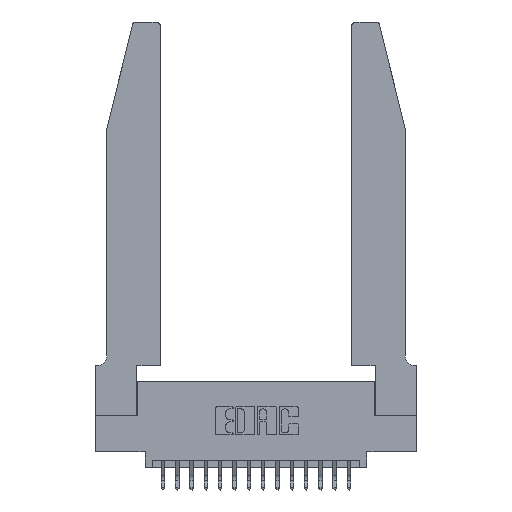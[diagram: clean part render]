
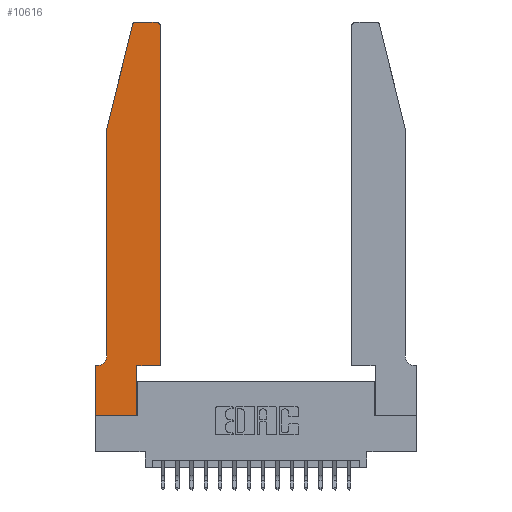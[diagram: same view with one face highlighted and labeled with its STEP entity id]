
A CAD part, top view. The second image highlights one B-rep face of the part: STEP entity #10616.
In plain terms, the highlighted planar face has unit normal (0, 0, 1).
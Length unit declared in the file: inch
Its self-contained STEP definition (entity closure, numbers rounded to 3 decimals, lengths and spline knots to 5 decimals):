
#74 = ORIENTED_EDGE ( 'NONE', *, *, #1063, .T. ) ;
#269 = DIRECTION ( 'NONE',  ( 0., 0., 1. ) ) ;
#299 = VECTOR ( 'NONE', #8002, 39.37008 ) ;
#442 = DIRECTION ( 'NONE',  ( -0.239, -0.971, 0. ) ) ;
#506 = CARTESIAN_POINT ( 'NONE',  ( 0.0755, 2., 0.37 ) ) ;
#681 = CARTESIAN_POINT ( 'NONE',  ( 0.0055, 0.35, 0.37 ) ) ;
#839 = VERTEX_POINT ( 'NONE', #16236 ) ;
#939 = CARTESIAN_POINT ( 'NONE',  ( 0., 0.35, 0.37 ) ) ;
#1063 = EDGE_CURVE ( 'NONE', #10182, #6074, #4686, .T. ) ;
#1089 = DIRECTION ( 'NONE',  ( -1., 0., 0. ) ) ;
#1125 = VECTOR ( 'NONE', #10548, 39.37008 ) ;
#1211 = CARTESIAN_POINT ( 'NONE',  ( 0.4505, 0.35, 0.37 ) ) ;
#1375 = EDGE_CURVE ( 'NONE', #12312, #8913, #15629, .T. ) ;
#1881 = VERTEX_POINT ( 'NONE', #1211 ) ;
#1940 = VECTOR ( 'NONE', #13911, 39.37008 ) ;
#2105 = AXIS2_PLACEMENT_3D ( 'NONE', #9655, #269, #11159 ) ;
#2196 = DIRECTION ( 'NONE',  ( 0., -1., 0. ) ) ;
#2913 = EDGE_CURVE ( 'NONE', #6074, #12196, #3329, .T. ) ;
#3329 = LINE ( 'NONE', #12933, #10999 ) ;
#4033 = CARTESIAN_POINT ( 'NONE',  ( 0.4205, 2.72, 0.37 ) ) ;
#4075 = LINE ( 'NONE', #17051, #299 ) ;
#4520 = DIRECTION ( 'NONE',  ( 0., 0., 1. ) ) ;
#4686 = LINE ( 'NONE', #16599, #12301 ) ;
#4693 = EDGE_LOOP ( 'NONE', ( #14164, #12269, #15600, #19391, #19447, #19095, #74, #7726, #13262, #17609, #11004, #9335 ) ) ;
#5027 = CARTESIAN_POINT ( 'NONE',  ( 0.2865, 0.35, 0.37 ) ) ;
#5591 = DIRECTION ( 'NONE',  ( 1., 0., 0. ) ) ;
#5601 = PLANE ( 'NONE',  #15617 ) ;
#5663 = LINE ( 'NONE', #18467, #1940 ) ;
#5685 = CARTESIAN_POINT ( 'NONE',  ( 0.2865, 0., 0.37 ) ) ;
#5727 = CARTESIAN_POINT ( 'NONE',  ( 0.4505, 0.35, 0.37 ) ) ;
#5868 = CIRCLE ( 'NONE', #13526, 0.03 ) ;
#6023 = CARTESIAN_POINT ( 'NONE',  ( 0.0755, 2., 0.37 ) ) ;
#6074 = VERTEX_POINT ( 'NONE', #13471 ) ;
#6077 = VECTOR ( 'NONE', #15677, 39.37008 ) ;
#6305 = EDGE_CURVE ( 'NONE', #1881, #10761, #5663, .T. ) ;
#7263 = VERTEX_POINT ( 'NONE', #681 ) ;
#7530 = EDGE_CURVE ( 'NONE', #15201, #16020, #12965, .T. ) ;
#7726 = ORIENTED_EDGE ( 'NONE', *, *, #2913, .T. ) ;
#8002 = DIRECTION ( 'NONE',  ( -1., 0., 0. ) ) ;
#8242 = EDGE_CURVE ( 'NONE', #12196, #8375, #17216, .T. ) ;
#8282 = VECTOR ( 'NONE', #442, 39.37008 ) ;
#8375 = VERTEX_POINT ( 'NONE', #14748 ) ;
#8755 = EDGE_CURVE ( 'NONE', #16020, #839, #12929, .T. ) ;
#8765 = DIRECTION ( 'NONE',  ( 1., 0., 0. ) ) ;
#8826 = DIRECTION ( 'NONE',  ( 1., 0., 0. ) ) ;
#8913 = VERTEX_POINT ( 'NONE', #9853 ) ;
#9111 = VECTOR ( 'NONE', #8826, 39.37008 ) ;
#9335 = ORIENTED_EDGE ( 'NONE', *, *, #16113, .T. ) ;
#9546 = EDGE_CURVE ( 'NONE', #7263, #10182, #4075, .T. ) ;
#9655 = CARTESIAN_POINT ( 'NONE',  ( 0.284, 2.72, 0.37 ) ) ;
#9821 = CARTESIAN_POINT ( 'NONE',  ( 0.0755, 2., 0.37 ) ) ;
#9853 = CARTESIAN_POINT ( 'NONE',  ( 0.0755, 0.42, 0.37 ) ) ;
#10182 = VERTEX_POINT ( 'NONE', #18460 ) ;
#10427 = DIRECTION ( 'NONE',  ( 0., 0., -1. ) ) ;
#10548 = DIRECTION ( 'NONE',  ( -1., 0., 0. ) ) ;
#10616 = ADVANCED_FACE ( 'NONE', ( #13607 ), #5601, .T. ) ;
#10761 = VERTEX_POINT ( 'NONE', #18506 ) ;
#10999 = VECTOR ( 'NONE', #8765, 39.37008 ) ;
#11004 = ORIENTED_EDGE ( 'NONE', *, *, #6305, .T. ) ;
#11102 = EDGE_CURVE ( 'NONE', #8375, #1881, #13111, .T. ) ;
#11159 = DIRECTION ( 'NONE',  ( 1., 0., 0. ) ) ;
#11789 = LINE ( 'NONE', #9821, #8282 ) ;
#12044 = VECTOR ( 'NONE', #2196, 39.37008 ) ;
#12196 = VERTEX_POINT ( 'NONE', #5685 ) ;
#12230 = AXIS2_PLACEMENT_3D ( 'NONE', #19437, #10427, #1089 ) ;
#12269 = ORIENTED_EDGE ( 'NONE', *, *, #8755, .T. ) ;
#12301 = VECTOR ( 'NONE', #14095, 39.37008 ) ;
#12312 = VERTEX_POINT ( 'NONE', #6023 ) ;
#12929 = CIRCLE ( 'NONE', #2105, 0.03 ) ;
#12933 = CARTESIAN_POINT ( 'NONE',  ( 0., 0., 0.37 ) ) ;
#12965 = LINE ( 'NONE', #19558, #1125 ) ;
#13111 = LINE ( 'NONE', #5727, #9111 ) ;
#13262 = ORIENTED_EDGE ( 'NONE', *, *, #8242, .T. ) ;
#13471 = CARTESIAN_POINT ( 'NONE',  ( 0., 0., 0.37 ) ) ;
#13526 = AXIS2_PLACEMENT_3D ( 'NONE', #4033, #14699, #5591 ) ;
#13607 = FACE_OUTER_BOUND ( 'NONE', #4693, .T. ) ;
#13911 = DIRECTION ( 'NONE',  ( 0., 1., 0. ) ) ;
#14095 = DIRECTION ( 'NONE',  ( 0., -1., 0. ) ) ;
#14164 = ORIENTED_EDGE ( 'NONE', *, *, #7530, .T. ) ;
#14699 = DIRECTION ( 'NONE',  ( 0., 0., 1. ) ) ;
#14748 = CARTESIAN_POINT ( 'NONE',  ( 0.2865, 0.35, 0.37 ) ) ;
#15164 = DIRECTION ( 'NONE',  ( 1., 0., 0. ) ) ;
#15201 = VERTEX_POINT ( 'NONE', #18287 ) ;
#15386 = CIRCLE ( 'NONE', #12230, 0.07 ) ;
#15590 = EDGE_CURVE ( 'NONE', #8913, #7263, #15386, .T. ) ;
#15600 = ORIENTED_EDGE ( 'NONE', *, *, #15965, .T. ) ;
#15617 = AXIS2_PLACEMENT_3D ( 'NONE', #939, #4520, #15164 ) ;
#15629 = LINE ( 'NONE', #506, #12044 ) ;
#15677 = DIRECTION ( 'NONE',  ( 0., 1., 0. ) ) ;
#15965 = EDGE_CURVE ( 'NONE', #839, #12312, #11789, .T. ) ;
#16020 = VERTEX_POINT ( 'NONE', #17464 ) ;
#16113 = EDGE_CURVE ( 'NONE', #10761, #15201, #5868, .T. ) ;
#16236 = CARTESIAN_POINT ( 'NONE',  ( 0.25487, 2.72718, 0.37 ) ) ;
#16599 = CARTESIAN_POINT ( 'NONE',  ( 0., 0., 0.37 ) ) ;
#17051 = CARTESIAN_POINT ( 'NONE',  ( 0.0755, 0.35, 0.37 ) ) ;
#17216 = LINE ( 'NONE', #5027, #6077 ) ;
#17464 = CARTESIAN_POINT ( 'NONE',  ( 0.284, 2.75, 0.37 ) ) ;
#17609 = ORIENTED_EDGE ( 'NONE', *, *, #11102, .T. ) ;
#18287 = CARTESIAN_POINT ( 'NONE',  ( 0.4205, 2.75, 0.37 ) ) ;
#18460 = CARTESIAN_POINT ( 'NONE',  ( 0., 0.35, 0.37 ) ) ;
#18467 = CARTESIAN_POINT ( 'NONE',  ( 0.4505, 0.35, 0.37 ) ) ;
#18506 = CARTESIAN_POINT ( 'NONE',  ( 0.4505, 2.72, 0.37 ) ) ;
#19095 = ORIENTED_EDGE ( 'NONE', *, *, #9546, .T. ) ;
#19391 = ORIENTED_EDGE ( 'NONE', *, *, #1375, .T. ) ;
#19437 = CARTESIAN_POINT ( 'NONE',  ( 0.0055, 0.42, 0.37 ) ) ;
#19447 = ORIENTED_EDGE ( 'NONE', *, *, #15590, .T. ) ;
#19558 = CARTESIAN_POINT ( 'NONE',  ( 0.2605, 2.75, 0.37 ) ) ;
